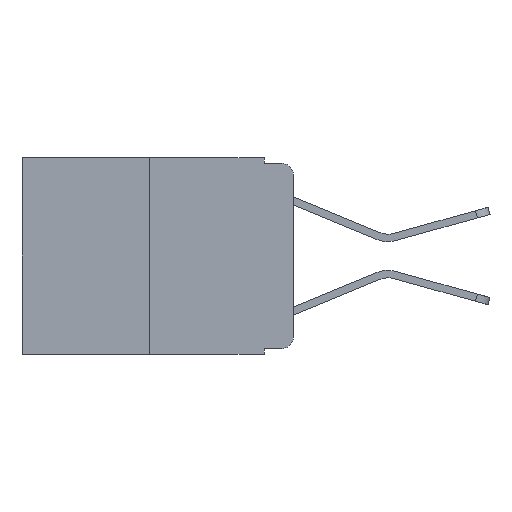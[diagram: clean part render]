
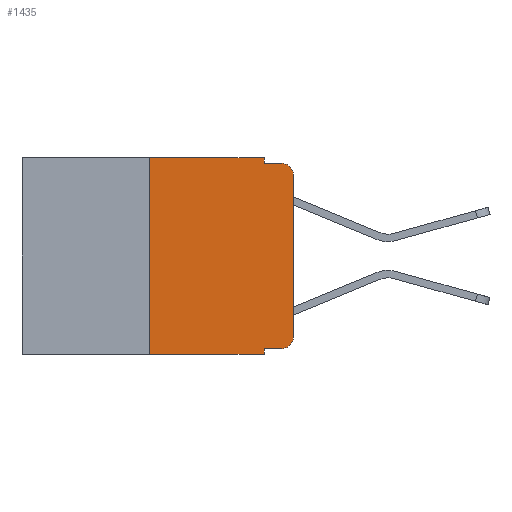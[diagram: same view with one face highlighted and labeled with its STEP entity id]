
A CAD part, left-side view. The second image highlights one B-rep face of the part: STEP entity #1435.
In plain terms, the highlighted planar face has unit normal (-1, 0, 0).
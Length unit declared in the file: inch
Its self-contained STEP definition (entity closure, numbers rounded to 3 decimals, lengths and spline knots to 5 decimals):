
#24 = DIRECTION ( 'NONE',  ( 0., 0., -1. ) ) ;
#604 = CARTESIAN_POINT ( 'NONE',  ( 0., 0.25, -0.343 ) ) ;
#994 = CARTESIAN_POINT ( 'NONE',  ( 0., 0.051, -0.333 ) ) ;
#1094 = EDGE_CURVE ( 'NONE', #3512, #2387, #5828, .T. ) ;
#1170 = CARTESIAN_POINT ( 'NONE',  ( 0., 0.473, 0. ) ) ;
#1435 = ADVANCED_FACE ( 'NONE', ( #4445 ), #9852, .F. ) ;
#1636 = EDGE_CURVE ( 'NONE', #5663, #4645, #10356, .T. ) ;
#1929 = DIRECTION ( 'NONE',  ( 0., 0., -1. ) ) ;
#2091 = EDGE_CURVE ( 'NONE', #10585, #6236, #10677, .T. ) ;
#2216 = EDGE_LOOP ( 'NONE', ( #13510, #12955, #13242, #9891, #8171, #8576, #5077, #8822, #11253, #4084 ) ) ;
#2245 = DIRECTION ( 'NONE',  ( 1., 0., 0. ) ) ;
#2260 = DIRECTION ( 'NONE',  ( 0., 0., -1. ) ) ;
#2387 = VERTEX_POINT ( 'NONE', #9001 ) ;
#2866 = LINE ( 'NONE', #7363, #9530 ) ;
#3018 = CARTESIAN_POINT ( 'NONE',  ( 0., 0.25, 0. ) ) ;
#3512 = VERTEX_POINT ( 'NONE', #994 ) ;
#3931 = CARTESIAN_POINT ( 'NONE',  ( 0., 0., 0. ) ) ;
#4084 = ORIENTED_EDGE ( 'NONE', *, *, #10283, .T. ) ;
#4139 = VECTOR ( 'NONE', #9790, 39.37008 ) ;
#4267 = CARTESIAN_POINT ( 'NONE',  ( 0., 0., -0.313 ) ) ;
#4445 = FACE_OUTER_BOUND ( 'NONE', #2216, .T. ) ;
#4487 = CARTESIAN_POINT ( 'NONE',  ( 0., 0.051, -0.01 ) ) ;
#4645 = VERTEX_POINT ( 'NONE', #4653 ) ;
#4653 = CARTESIAN_POINT ( 'NONE',  ( 0., 0., -0.03 ) ) ;
#4941 = CARTESIAN_POINT ( 'NONE',  ( 0., 0.051, -0.343 ) ) ;
#5077 = ORIENTED_EDGE ( 'NONE', *, *, #2091, .T. ) ;
#5148 = CARTESIAN_POINT ( 'NONE',  ( 0., 0.051, -0.01 ) ) ;
#5509 = EDGE_CURVE ( 'NONE', #11151, #12007, #2866, .T. ) ;
#5663 = VERTEX_POINT ( 'NONE', #4267 ) ;
#5828 = LINE ( 'NONE', #13366, #8759 ) ;
#6236 = VERTEX_POINT ( 'NONE', #4941 ) ;
#6503 = LINE ( 'NONE', #4487, #8491 ) ;
#6616 = DIRECTION ( 'NONE',  ( -1., 0., 0. ) ) ;
#6682 = AXIS2_PLACEMENT_3D ( 'NONE', #9639, #13993, #12921 ) ;
#6731 = CARTESIAN_POINT ( 'NONE',  ( 0., 0.25, 0. ) ) ;
#7363 = CARTESIAN_POINT ( 'NONE',  ( 0., 0.051, 0. ) ) ;
#7555 = LINE ( 'NONE', #14136, #4139 ) ;
#7663 = VECTOR ( 'NONE', #13624, 39.37008 ) ;
#7765 = CARTESIAN_POINT ( 'NONE',  ( 0., 0.02, -0.03 ) ) ;
#8064 = VERTEX_POINT ( 'NONE', #10297 ) ;
#8171 = ORIENTED_EDGE ( 'NONE', *, *, #11193, .F. ) ;
#8234 = EDGE_CURVE ( 'NONE', #10585, #10645, #8952, .T. ) ;
#8491 = VECTOR ( 'NONE', #12181, 39.37008 ) ;
#8576 = ORIENTED_EDGE ( 'NONE', *, *, #8234, .F. ) ;
#8759 = VECTOR ( 'NONE', #13292, 39.37008 ) ;
#8802 = DIRECTION ( 'NONE',  ( 0., 0., 1. ) ) ;
#8822 = ORIENTED_EDGE ( 'NONE', *, *, #11629, .F. ) ;
#8952 = LINE ( 'NONE', #6731, #13513 ) ;
#9001 = CARTESIAN_POINT ( 'NONE',  ( 0., 0.02, -0.333 ) ) ;
#9489 = EDGE_CURVE ( 'NONE', #12007, #8064, #6503, .T. ) ;
#9530 = VECTOR ( 'NONE', #1929, 39.37008 ) ;
#9639 = CARTESIAN_POINT ( 'NONE',  ( 0., 0.02, -0.313 ) ) ;
#9790 = DIRECTION ( 'NONE',  ( 0., 0., -1. ) ) ;
#9808 = CARTESIAN_POINT ( 'NONE',  ( 0., 0.473, 0. ) ) ;
#9852 = PLANE ( 'NONE',  #13426 ) ;
#9885 = DIRECTION ( 'NONE',  ( 0., -1., 0. ) ) ;
#9891 = ORIENTED_EDGE ( 'NONE', *, *, #5509, .F. ) ;
#10283 = EDGE_CURVE ( 'NONE', #2387, #5663, #14001, .T. ) ;
#10297 = CARTESIAN_POINT ( 'NONE',  ( 0., 0.02, -0.01 ) ) ;
#10356 = LINE ( 'NONE', #3931, #7663 ) ;
#10585 = VERTEX_POINT ( 'NONE', #604 ) ;
#10645 = VERTEX_POINT ( 'NONE', #3018 ) ;
#10677 = LINE ( 'NONE', #12661, #13259 ) ;
#11151 = VERTEX_POINT ( 'NONE', #13946 ) ;
#11193 = EDGE_CURVE ( 'NONE', #10645, #11151, #12944, .T. ) ;
#11253 = ORIENTED_EDGE ( 'NONE', *, *, #1094, .T. ) ;
#11556 = CIRCLE ( 'NONE', #13606, 0.02 ) ;
#11629 = EDGE_CURVE ( 'NONE', #3512, #6236, #7555, .T. ) ;
#12007 = VERTEX_POINT ( 'NONE', #5148 ) ;
#12181 = DIRECTION ( 'NONE',  ( 0., -1., 0. ) ) ;
#12661 = CARTESIAN_POINT ( 'NONE',  ( 0., 0.473, -0.343 ) ) ;
#12921 = DIRECTION ( 'NONE',  ( 0., 0., -1. ) ) ;
#12944 = LINE ( 'NONE', #9808, #13573 ) ;
#12955 = ORIENTED_EDGE ( 'NONE', *, *, #14083, .T. ) ;
#13242 = ORIENTED_EDGE ( 'NONE', *, *, #9489, .F. ) ;
#13259 = VECTOR ( 'NONE', #13800, 39.37008 ) ;
#13292 = DIRECTION ( 'NONE',  ( 0., -1., 0. ) ) ;
#13366 = CARTESIAN_POINT ( 'NONE',  ( 0., 0.051, -0.333 ) ) ;
#13426 = AXIS2_PLACEMENT_3D ( 'NONE', #1170, #2245, #24 ) ;
#13510 = ORIENTED_EDGE ( 'NONE', *, *, #1636, .T. ) ;
#13513 = VECTOR ( 'NONE', #8802, 39.37008 ) ;
#13573 = VECTOR ( 'NONE', #9885, 39.37008 ) ;
#13606 = AXIS2_PLACEMENT_3D ( 'NONE', #7765, #6616, #2260 ) ;
#13624 = DIRECTION ( 'NONE',  ( 0., 0., 1. ) ) ;
#13800 = DIRECTION ( 'NONE',  ( 0., -1., 0. ) ) ;
#13946 = CARTESIAN_POINT ( 'NONE',  ( 0., 0.051, 0. ) ) ;
#13993 = DIRECTION ( 'NONE',  ( -1., 0., 0. ) ) ;
#14001 = CIRCLE ( 'NONE', #6682, 0.02 ) ;
#14083 = EDGE_CURVE ( 'NONE', #4645, #8064, #11556, .T. ) ;
#14136 = CARTESIAN_POINT ( 'NONE',  ( 0., 0.051, 0. ) ) ;
